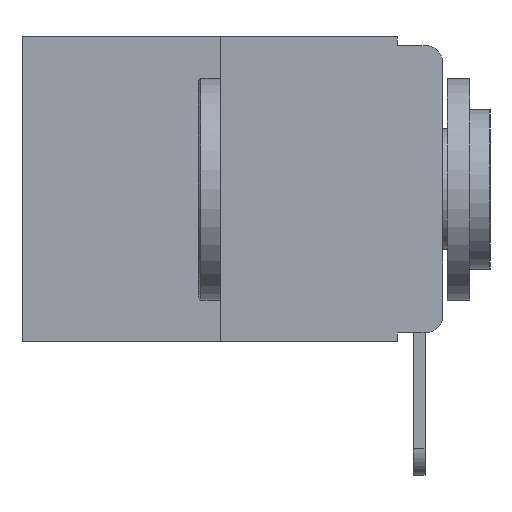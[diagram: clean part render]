
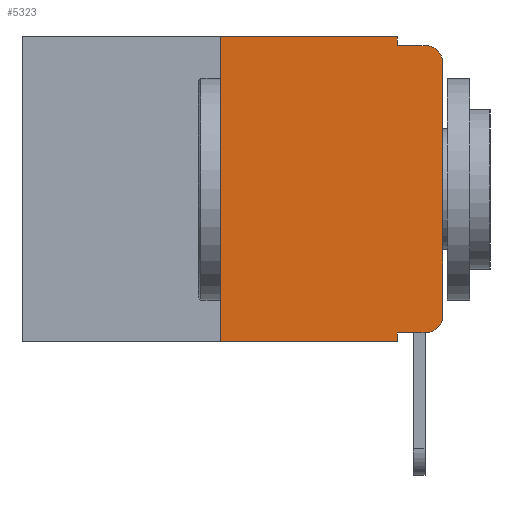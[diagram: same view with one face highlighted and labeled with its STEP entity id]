
A CAD part, left-side view. The second image highlights one B-rep face of the part: STEP entity #5323.
In plain terms, the highlighted planar face has unit normal (-1, 0, 0).
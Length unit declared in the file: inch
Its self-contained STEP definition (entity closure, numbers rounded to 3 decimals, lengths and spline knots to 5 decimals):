
#36 = VECTOR ( 'NONE', #9678, 39.37008 ) ;
#91 = CARTESIAN_POINT ( 'NONE',  ( 0., 0.25, -0.343 ) ) ;
#120 = VERTEX_POINT ( 'NONE', #2068 ) ;
#236 = EDGE_CURVE ( 'NONE', #6798, #12186, #6280, .T. ) ;
#298 = ORIENTED_EDGE ( 'NONE', *, *, #7794, .T. ) ;
#367 = ORIENTED_EDGE ( 'NONE', *, *, #8536, .T. ) ;
#708 = VECTOR ( 'NONE', #10730, 39.37008 ) ;
#720 = DIRECTION ( 'NONE',  ( -1., 0., 0. ) ) ;
#760 = ORIENTED_EDGE ( 'NONE', *, *, #1631, .T. ) ;
#802 = DIRECTION ( 'NONE',  ( 0., 0., -1. ) ) ;
#1017 = VECTOR ( 'NONE', #1734, 39.37008 ) ;
#1065 = FACE_OUTER_BOUND ( 'NONE', #5337, .T. ) ;
#1193 = VERTEX_POINT ( 'NONE', #2916 ) ;
#1224 = VECTOR ( 'NONE', #9328, 39.37008 ) ;
#1423 = DIRECTION ( 'NONE',  ( 0., -1., 0. ) ) ;
#1631 = EDGE_CURVE ( 'NONE', #120, #2543, #7395, .T. ) ;
#1734 = DIRECTION ( 'NONE',  ( 0., -1., 0. ) ) ;
#1915 = ORIENTED_EDGE ( 'NONE', *, *, #2115, .F. ) ;
#2059 = VERTEX_POINT ( 'NONE', #5912 ) ;
#2068 = CARTESIAN_POINT ( 'NONE',  ( 0., 0.02, -0.333 ) ) ;
#2115 = EDGE_CURVE ( 'NONE', #2059, #8087, #2753, .T. ) ;
#2491 = DIRECTION ( 'NONE',  ( 0., 0., 1. ) ) ;
#2543 = VERTEX_POINT ( 'NONE', #8990 ) ;
#2753 = LINE ( 'NONE', #8277, #9886 ) ;
#2916 = CARTESIAN_POINT ( 'NONE',  ( 0., 0.051, -0.333 ) ) ;
#3009 = AXIS2_PLACEMENT_3D ( 'NONE', #10924, #720, #802 ) ;
#3076 = EDGE_CURVE ( 'NONE', #1193, #120, #7682, .T. ) ;
#3373 = VERTEX_POINT ( 'NONE', #7472 ) ;
#3413 = CARTESIAN_POINT ( 'NONE',  ( 0., 0., 0. ) ) ;
#3433 = AXIS2_PLACEMENT_3D ( 'NONE', #10932, #12912, #11971 ) ;
#4430 = PLANE ( 'NONE',  #12493 ) ;
#5227 = LINE ( 'NONE', #6570, #10806 ) ;
#5232 = DIRECTION ( 'NONE',  ( 0., 0., -1. ) ) ;
#5323 = ADVANCED_FACE ( 'NONE', ( #1065 ), #4430, .F. ) ;
#5337 = EDGE_LOOP ( 'NONE', ( #367, #7352, #12952, #1915, #6444, #6390, #298, #9779, #12680, #760 ) ) ;
#5348 = CARTESIAN_POINT ( 'NONE',  ( 0., 0.051, -0.01 ) ) ;
#5738 = LINE ( 'NONE', #3413, #36 ) ;
#5820 = LINE ( 'NONE', #5348, #1224 ) ;
#5912 = CARTESIAN_POINT ( 'NONE',  ( 0., 0.051, 0. ) ) ;
#6220 = VERTEX_POINT ( 'NONE', #91 ) ;
#6280 = CIRCLE ( 'NONE', #3433, 0.02 ) ;
#6390 = ORIENTED_EDGE ( 'NONE', *, *, #9054, .F. ) ;
#6444 = ORIENTED_EDGE ( 'NONE', *, *, #9727, .F. ) ;
#6478 = EDGE_CURVE ( 'NONE', #1193, #12831, #9426, .T. ) ;
#6503 = DIRECTION ( 'NONE',  ( 0., 0., -1. ) ) ;
#6570 = CARTESIAN_POINT ( 'NONE',  ( 0., 0.473, 0. ) ) ;
#6798 = VERTEX_POINT ( 'NONE', #12328 ) ;
#7352 = ORIENTED_EDGE ( 'NONE', *, *, #236, .T. ) ;
#7395 = CIRCLE ( 'NONE', #3009, 0.02 ) ;
#7472 = CARTESIAN_POINT ( 'NONE',  ( 0., 0.25, 0. ) ) ;
#7662 = CARTESIAN_POINT ( 'NONE',  ( 0., 0.473, -0.343 ) ) ;
#7682 = LINE ( 'NONE', #11882, #1017 ) ;
#7794 = EDGE_CURVE ( 'NONE', #6220, #12831, #8804, .T. ) ;
#7975 = LINE ( 'NONE', #9496, #10819 ) ;
#8087 = VERTEX_POINT ( 'NONE', #10266 ) ;
#8277 = CARTESIAN_POINT ( 'NONE',  ( 0., 0.051, 0. ) ) ;
#8536 = EDGE_CURVE ( 'NONE', #2543, #6798, #5738, .T. ) ;
#8623 = CARTESIAN_POINT ( 'NONE',  ( 0., 0.051, -0.343 ) ) ;
#8635 = CARTESIAN_POINT ( 'NONE',  ( 0., 0.02, -0.01 ) ) ;
#8804 = LINE ( 'NONE', #7662, #11670 ) ;
#8990 = CARTESIAN_POINT ( 'NONE',  ( 0., 0., -0.313 ) ) ;
#9054 = EDGE_CURVE ( 'NONE', #6220, #3373, #7975, .T. ) ;
#9328 = DIRECTION ( 'NONE',  ( 0., -1., 0. ) ) ;
#9426 = LINE ( 'NONE', #10865, #708 ) ;
#9496 = CARTESIAN_POINT ( 'NONE',  ( 0., 0.25, 0. ) ) ;
#9678 = DIRECTION ( 'NONE',  ( 0., 0., 1. ) ) ;
#9727 = EDGE_CURVE ( 'NONE', #3373, #2059, #5227, .T. ) ;
#9779 = ORIENTED_EDGE ( 'NONE', *, *, #6478, .F. ) ;
#9886 = VECTOR ( 'NONE', #5232, 39.37008 ) ;
#10266 = CARTESIAN_POINT ( 'NONE',  ( 0., 0.051, -0.01 ) ) ;
#10494 = DIRECTION ( 'NONE',  ( 1., 0., 0. ) ) ;
#10622 = CARTESIAN_POINT ( 'NONE',  ( 0., 0.473, 0. ) ) ;
#10730 = DIRECTION ( 'NONE',  ( 0., 0., -1. ) ) ;
#10806 = VECTOR ( 'NONE', #1423, 39.37008 ) ;
#10819 = VECTOR ( 'NONE', #2491, 39.37008 ) ;
#10865 = CARTESIAN_POINT ( 'NONE',  ( 0., 0.051, 0. ) ) ;
#10924 = CARTESIAN_POINT ( 'NONE',  ( 0., 0.02, -0.313 ) ) ;
#10932 = CARTESIAN_POINT ( 'NONE',  ( 0., 0.02, -0.03 ) ) ;
#11460 = EDGE_CURVE ( 'NONE', #8087, #12186, #5820, .T. ) ;
#11670 = VECTOR ( 'NONE', #12776, 39.37008 ) ;
#11882 = CARTESIAN_POINT ( 'NONE',  ( 0., 0.051, -0.333 ) ) ;
#11971 = DIRECTION ( 'NONE',  ( 0., 0., -1. ) ) ;
#12186 = VERTEX_POINT ( 'NONE', #8635 ) ;
#12328 = CARTESIAN_POINT ( 'NONE',  ( 0., 0., -0.03 ) ) ;
#12493 = AXIS2_PLACEMENT_3D ( 'NONE', #10622, #10494, #6503 ) ;
#12680 = ORIENTED_EDGE ( 'NONE', *, *, #3076, .T. ) ;
#12776 = DIRECTION ( 'NONE',  ( 0., -1., 0. ) ) ;
#12831 = VERTEX_POINT ( 'NONE', #8623 ) ;
#12912 = DIRECTION ( 'NONE',  ( -1., 0., 0. ) ) ;
#12952 = ORIENTED_EDGE ( 'NONE', *, *, #11460, .F. ) ;
